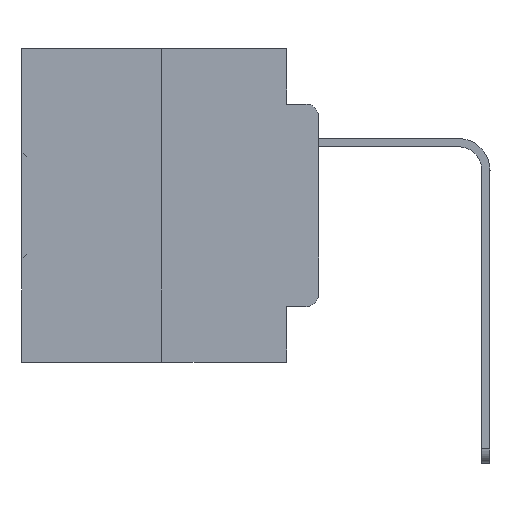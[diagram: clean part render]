
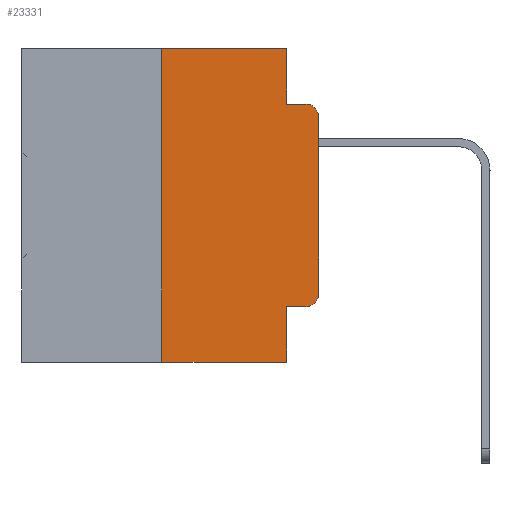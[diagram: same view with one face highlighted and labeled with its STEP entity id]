
A CAD part, left-side view. The second image highlights one B-rep face of the part: STEP entity #23331.
In plain terms, the highlighted planar face has unit normal (-1, 0, 0).
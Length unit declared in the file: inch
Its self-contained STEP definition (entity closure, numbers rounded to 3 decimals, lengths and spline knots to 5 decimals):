
#129 = VECTOR ( 'NONE', #23781, 39.37008 ) ;
#283 = LINE ( 'NONE', #25628, #6576 ) ;
#1124 = CARTESIAN_POINT ( 'NONE',  ( 0., 0.051, -0.4115 ) ) ;
#1453 = DIRECTION ( 'NONE',  ( -1., 0., 0. ) ) ;
#1511 = DIRECTION ( 'NONE',  ( 0., 0., -1. ) ) ;
#1677 = DIRECTION ( 'NONE',  ( 1., 0., 0. ) ) ;
#2063 = DIRECTION ( 'NONE',  ( 0., 0., 1. ) ) ;
#2313 = DIRECTION ( 'NONE',  ( 0., -1., 0. ) ) ;
#2675 = LINE ( 'NONE', #19270, #15904 ) ;
#2698 = EDGE_CURVE ( 'NONE', #32271, #16226, #2675, .T. ) ;
#4314 = EDGE_CURVE ( 'NONE', #23044, #25387, #283, .T. ) ;
#4486 = VECTOR ( 'NONE', #19794, 39.37008 ) ;
#4614 = CARTESIAN_POINT ( 'NONE',  ( 0., 0.02, -0.4115 ) ) ;
#5087 = LINE ( 'NONE', #8546, #11290 ) ;
#5892 = AXIS2_PLACEMENT_3D ( 'NONE', #16838, #1677, #19148 ) ;
#6074 = VERTEX_POINT ( 'NONE', #24341 ) ;
#6165 = LINE ( 'NONE', #6573, #24924 ) ;
#6573 = CARTESIAN_POINT ( 'NONE',  ( 0., 0., 0. ) ) ;
#6576 = VECTOR ( 'NONE', #18171, 39.37008 ) ;
#7375 = VECTOR ( 'NONE', #8243, 39.37008 ) ;
#7541 = EDGE_CURVE ( 'NONE', #9678, #25387, #16401, .T. ) ;
#8243 = DIRECTION ( 'NONE',  ( 0., 0., 1. ) ) ;
#8253 = CARTESIAN_POINT ( 'NONE',  ( 0., 0.051, -0.0885 ) ) ;
#8546 = CARTESIAN_POINT ( 'NONE',  ( 0., 0.051, 0. ) ) ;
#8969 = DIRECTION ( 'NONE',  ( -1., 0., 0. ) ) ;
#9239 = CARTESIAN_POINT ( 'NONE',  ( 0., 0.02, -0.0885 ) ) ;
#9270 = CARTESIAN_POINT ( 'NONE',  ( 0., 0., -0.1085 ) ) ;
#9678 = VERTEX_POINT ( 'NONE', #9270 ) ;
#9680 = CARTESIAN_POINT ( 'NONE',  ( 0., 0.25, 0. ) ) ;
#10742 = VERTEX_POINT ( 'NONE', #4614 ) ;
#11079 = LINE ( 'NONE', #14217, #4486 ) ;
#11242 = FACE_OUTER_BOUND ( 'NONE', #27023, .T. ) ;
#11271 = DIRECTION ( 'NONE',  ( 0., 0., -1. ) ) ;
#11290 = VECTOR ( 'NONE', #15703, 39.37008 ) ;
#11607 = ORIENTED_EDGE ( 'NONE', *, *, #20173, .F. ) ;
#12000 = EDGE_CURVE ( 'NONE', #6074, #32271, #19860, .T. ) ;
#12892 = EDGE_CURVE ( 'NONE', #19168, #9678, #6165, .T. ) ;
#14003 = PLANE ( 'NONE',  #5892 ) ;
#14217 = CARTESIAN_POINT ( 'NONE',  ( 0., 0.473, -0.5 ) ) ;
#14339 = DIRECTION ( 'NONE',  ( 0., -1., 0. ) ) ;
#14416 = EDGE_CURVE ( 'NONE', #19821, #10742, #30679, .T. ) ;
#14933 = CARTESIAN_POINT ( 'NONE',  ( 0., 0.051, -0.4115 ) ) ;
#15703 = DIRECTION ( 'NONE',  ( 0., 0., -1. ) ) ;
#15904 = VECTOR ( 'NONE', #14339, 39.37008 ) ;
#16226 = VERTEX_POINT ( 'NONE', #24600 ) ;
#16401 = CIRCLE ( 'NONE', #16618, 0.02 ) ;
#16504 = CARTESIAN_POINT ( 'NONE',  ( 0., 0.02, -0.3915 ) ) ;
#16618 = AXIS2_PLACEMENT_3D ( 'NONE', #21394, #8969, #1511 ) ;
#16838 = CARTESIAN_POINT ( 'NONE',  ( 0., 0.473, 0. ) ) ;
#17057 = ORIENTED_EDGE ( 'NONE', *, *, #30452, .F. ) ;
#18171 = DIRECTION ( 'NONE',  ( 0., -1., 0. ) ) ;
#18394 = ORIENTED_EDGE ( 'NONE', *, *, #25226, .T. ) ;
#18502 = VECTOR ( 'NONE', #2313, 39.37008 ) ;
#18743 = CARTESIAN_POINT ( 'NONE',  ( 0., 0.051, -0.5 ) ) ;
#18875 = ORIENTED_EDGE ( 'NONE', *, *, #14416, .T. ) ;
#19148 = DIRECTION ( 'NONE',  ( 0., 0., -1. ) ) ;
#19168 = VERTEX_POINT ( 'NONE', #29491 ) ;
#19270 = CARTESIAN_POINT ( 'NONE',  ( 0., 0.473, 0. ) ) ;
#19794 = DIRECTION ( 'NONE',  ( 0., -1., 0. ) ) ;
#19821 = VERTEX_POINT ( 'NONE', #1124 ) ;
#19860 = LINE ( 'NONE', #25605, #7375 ) ;
#19966 = ORIENTED_EDGE ( 'NONE', *, *, #29516, .T. ) ;
#20173 = EDGE_CURVE ( 'NONE', #16226, #23044, #5087, .T. ) ;
#21394 = CARTESIAN_POINT ( 'NONE',  ( 0., 0.02, -0.1085 ) ) ;
#22792 = ORIENTED_EDGE ( 'NONE', *, *, #2698, .F. ) ;
#23044 = VERTEX_POINT ( 'NONE', #8253 ) ;
#23045 = AXIS2_PLACEMENT_3D ( 'NONE', #16504, #1453, #11271 ) ;
#23331 = ADVANCED_FACE ( 'NONE', ( #11242 ), #14003, .F. ) ;
#23781 = DIRECTION ( 'NONE',  ( 0., 0., -1. ) ) ;
#24148 = ORIENTED_EDGE ( 'NONE', *, *, #12000, .F. ) ;
#24341 = CARTESIAN_POINT ( 'NONE',  ( 0., 0.25, -0.5 ) ) ;
#24552 = ORIENTED_EDGE ( 'NONE', *, *, #4314, .F. ) ;
#24600 = CARTESIAN_POINT ( 'NONE',  ( 0., 0.051, 0. ) ) ;
#24924 = VECTOR ( 'NONE', #2063, 39.37008 ) ;
#25226 = EDGE_CURVE ( 'NONE', #10742, #19168, #25248, .T. ) ;
#25248 = CIRCLE ( 'NONE', #23045, 0.02 ) ;
#25387 = VERTEX_POINT ( 'NONE', #9239 ) ;
#25605 = CARTESIAN_POINT ( 'NONE',  ( 0., 0.25, 0. ) ) ;
#25628 = CARTESIAN_POINT ( 'NONE',  ( 0., 0.051, -0.0885 ) ) ;
#27023 = EDGE_LOOP ( 'NONE', ( #30601, #32314, #24552, #11607, #22792, #24148, #19966, #17057, #18875, #18394 ) ) ;
#28286 = LINE ( 'NONE', #28604, #129 ) ;
#28604 = CARTESIAN_POINT ( 'NONE',  ( 0., 0.051, 0. ) ) ;
#29491 = CARTESIAN_POINT ( 'NONE',  ( 0., 0., -0.3915 ) ) ;
#29516 = EDGE_CURVE ( 'NONE', #6074, #30479, #11079, .T. ) ;
#30452 = EDGE_CURVE ( 'NONE', #19821, #30479, #28286, .T. ) ;
#30479 = VERTEX_POINT ( 'NONE', #18743 ) ;
#30601 = ORIENTED_EDGE ( 'NONE', *, *, #12892, .T. ) ;
#30679 = LINE ( 'NONE', #14933, #18502 ) ;
#32271 = VERTEX_POINT ( 'NONE', #9680 ) ;
#32314 = ORIENTED_EDGE ( 'NONE', *, *, #7541, .T. ) ;
